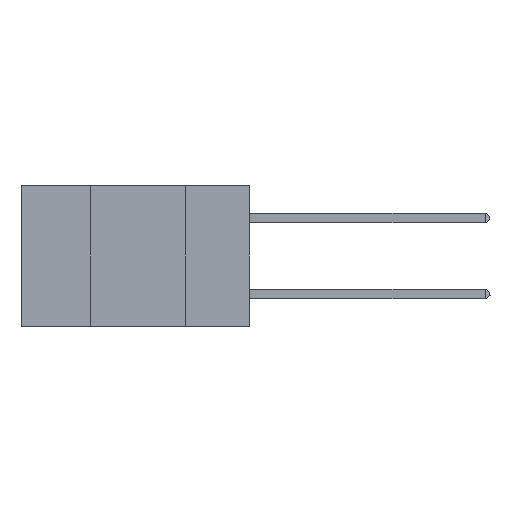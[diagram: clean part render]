
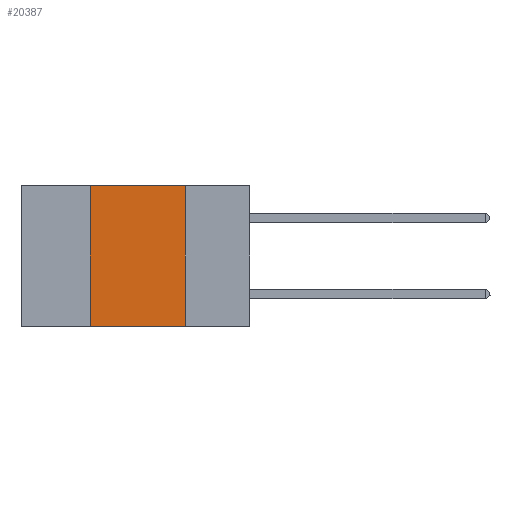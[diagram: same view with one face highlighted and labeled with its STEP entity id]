
A CAD part, left-side view. The second image highlights one B-rep face of the part: STEP entity #20387.
In plain terms, the highlighted planar face has unit normal (-1, 0, 0).
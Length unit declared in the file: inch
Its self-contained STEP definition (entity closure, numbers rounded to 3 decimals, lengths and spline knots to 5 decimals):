
#187 = EDGE_CURVE ( 'NONE', #9391, #21772, #16927, .T. ) ;
#1583 = LINE ( 'NONE', #18462, #14040 ) ;
#1863 = VECTOR ( 'NONE', #13137, 39.37008 ) ;
#4333 = CARTESIAN_POINT ( 'NONE',  ( 0., 0.17, 0. ) ) ;
#6382 = DIRECTION ( 'NONE',  ( 1., 0., 0. ) ) ;
#6555 = VECTOR ( 'NONE', #14581, 39.37008 ) ;
#7797 = PLANE ( 'NONE',  #15382 ) ;
#7846 = CARTESIAN_POINT ( 'NONE',  ( 0., 0.17, 0. ) ) ;
#7977 = LINE ( 'NONE', #10764, #19960 ) ;
#8034 = ORIENTED_EDGE ( 'NONE', *, *, #187, .F. ) ;
#8209 = FACE_OUTER_BOUND ( 'NONE', #20781, .T. ) ;
#9391 = VERTEX_POINT ( 'NONE', #4333 ) ;
#9821 = LINE ( 'NONE', #11606, #1863 ) ;
#10764 = CARTESIAN_POINT ( 'NONE',  ( 0., 0.6, 0. ) ) ;
#11606 = CARTESIAN_POINT ( 'NONE',  ( 0., 0.42, 0. ) ) ;
#11950 = EDGE_CURVE ( 'NONE', #13013, #19599, #9821, .T. ) ;
#11963 = DIRECTION ( 'NONE',  ( 0., 0., -1. ) ) ;
#12553 = CARTESIAN_POINT ( 'NONE',  ( 0., 0.17, -0.37 ) ) ;
#13013 = VERTEX_POINT ( 'NONE', #18315 ) ;
#13137 = DIRECTION ( 'NONE',  ( 0., 0., 1. ) ) ;
#13796 = DIRECTION ( 'NONE',  ( 0., -1., 0. ) ) ;
#14040 = VECTOR ( 'NONE', #21825, 39.37008 ) ;
#14581 = DIRECTION ( 'NONE',  ( 0., 0., -1. ) ) ;
#15382 = AXIS2_PLACEMENT_3D ( 'NONE', #18082, #6382, #11963 ) ;
#15539 = EDGE_CURVE ( 'NONE', #19599, #9391, #7977, .T. ) ;
#16927 = LINE ( 'NONE', #7846, #6555 ) ;
#17092 = ORIENTED_EDGE ( 'NONE', *, *, #19853, .T. ) ;
#17501 = CARTESIAN_POINT ( 'NONE',  ( 0., 0.42, 0. ) ) ;
#18082 = CARTESIAN_POINT ( 'NONE',  ( 0., 0.6, 0. ) ) ;
#18315 = CARTESIAN_POINT ( 'NONE',  ( 0., 0.42, -0.37 ) ) ;
#18462 = CARTESIAN_POINT ( 'NONE',  ( 0., 0.6, -0.37 ) ) ;
#19599 = VERTEX_POINT ( 'NONE', #17501 ) ;
#19853 = EDGE_CURVE ( 'NONE', #13013, #21772, #1583, .T. ) ;
#19960 = VECTOR ( 'NONE', #13796, 39.37008 ) ;
#20387 = ADVANCED_FACE ( 'NONE', ( #8209 ), #7797, .F. ) ;
#20781 = EDGE_LOOP ( 'NONE', ( #8034, #21762, #21000, #17092 ) ) ;
#21000 = ORIENTED_EDGE ( 'NONE', *, *, #11950, .F. ) ;
#21762 = ORIENTED_EDGE ( 'NONE', *, *, #15539, .F. ) ;
#21772 = VERTEX_POINT ( 'NONE', #12553 ) ;
#21825 = DIRECTION ( 'NONE',  ( 0., -1., 0. ) ) ;
